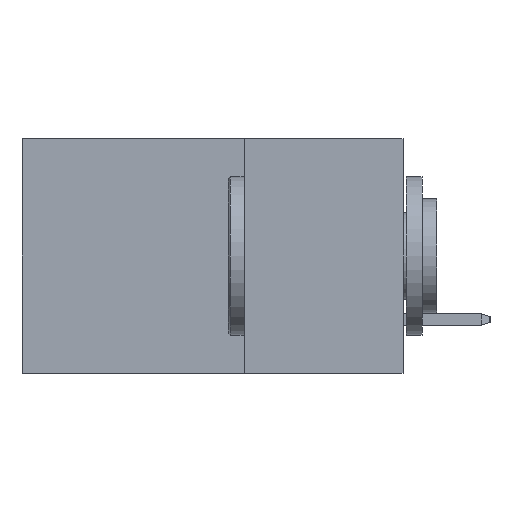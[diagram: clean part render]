
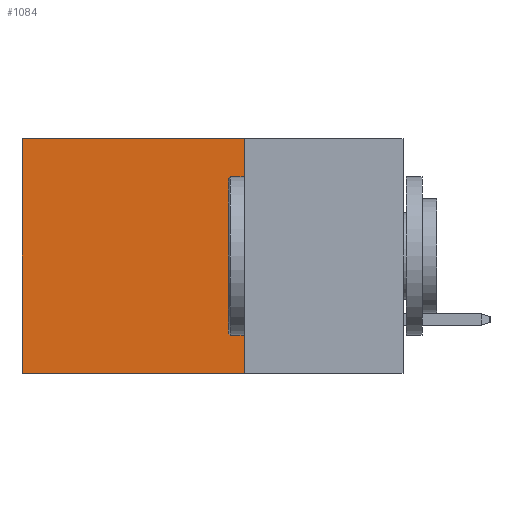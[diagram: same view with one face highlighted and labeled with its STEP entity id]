
A CAD part, left-side view. The second image highlights one B-rep face of the part: STEP entity #1084.
In plain terms, the highlighted planar face has unit normal (-1, 0, 0).
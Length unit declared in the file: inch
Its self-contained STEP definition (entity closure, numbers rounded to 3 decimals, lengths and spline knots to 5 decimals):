
#391 = AXIS2_PLACEMENT_3D ( 'NONE', #1517, #6967, #6068 ) ;
#585 = VERTEX_POINT ( 'NONE', #7213 ) ;
#739 = CARTESIAN_POINT ( 'NONE',  ( 0.2875, 0.6, 0. ) ) ;
#1084 = ADVANCED_FACE ( 'NONE', ( #11566 ), #3276, .F. ) ;
#1517 = CARTESIAN_POINT ( 'NONE',  ( 0.2875, 0.25, 0. ) ) ;
#2799 = ORIENTED_EDGE ( 'NONE', *, *, #11179, .F. ) ;
#3276 = PLANE ( 'NONE',  #391 ) ;
#3330 = LINE ( 'NONE', #739, #11479 ) ;
#3547 = ORIENTED_EDGE ( 'NONE', *, *, #5794, .T. ) ;
#3858 = EDGE_LOOP ( 'NONE', ( #3547, #7977, #2799, #9651 ) ) ;
#4308 = VECTOR ( 'NONE', #11584, 39.37008 ) ;
#4541 = CARTESIAN_POINT ( 'NONE',  ( 0.2875, 0.25, -0.37 ) ) ;
#5175 = LINE ( 'NONE', #6020, #4308 ) ;
#5554 = CARTESIAN_POINT ( 'NONE',  ( 0.2875, 0.6, -0.37 ) ) ;
#5647 = CARTESIAN_POINT ( 'NONE',  ( 0.2875, 0.25, -0.37 ) ) ;
#5794 = EDGE_CURVE ( 'NONE', #585, #6385, #3330, .T. ) ;
#5885 = EDGE_CURVE ( 'NONE', #6714, #6385, #7479, .T. ) ;
#6020 = CARTESIAN_POINT ( 'NONE',  ( 0.2875, 0.25, 0. ) ) ;
#6056 = VECTOR ( 'NONE', #10799, 39.37008 ) ;
#6068 = DIRECTION ( 'NONE',  ( 0., 0., -1. ) ) ;
#6274 = CARTESIAN_POINT ( 'NONE',  ( 0.2875, 0.25, 0. ) ) ;
#6385 = VERTEX_POINT ( 'NONE', #5554 ) ;
#6714 = VERTEX_POINT ( 'NONE', #5647 ) ;
#6967 = DIRECTION ( 'NONE',  ( 1., 0., 0. ) ) ;
#7213 = CARTESIAN_POINT ( 'NONE',  ( 0.2875, 0.6, 0. ) ) ;
#7229 = LINE ( 'NONE', #6274, #6056 ) ;
#7479 = LINE ( 'NONE', #4541, #8343 ) ;
#7977 = ORIENTED_EDGE ( 'NONE', *, *, #5885, .F. ) ;
#8343 = VECTOR ( 'NONE', #10206, 39.37008 ) ;
#9651 = ORIENTED_EDGE ( 'NONE', *, *, #11225, .T. ) ;
#9866 = VERTEX_POINT ( 'NONE', #11470 ) ;
#10206 = DIRECTION ( 'NONE',  ( 0., 1., 0. ) ) ;
#10799 = DIRECTION ( 'NONE',  ( 0., 1., 0. ) ) ;
#10899 = DIRECTION ( 'NONE',  ( 0., 0., -1. ) ) ;
#11179 = EDGE_CURVE ( 'NONE', #9866, #6714, #5175, .T. ) ;
#11225 = EDGE_CURVE ( 'NONE', #9866, #585, #7229, .T. ) ;
#11470 = CARTESIAN_POINT ( 'NONE',  ( 0.2875, 0.25, 0. ) ) ;
#11479 = VECTOR ( 'NONE', #10899, 39.37008 ) ;
#11566 = FACE_OUTER_BOUND ( 'NONE', #3858, .T. ) ;
#11584 = DIRECTION ( 'NONE',  ( 0., 0., -1. ) ) ;
